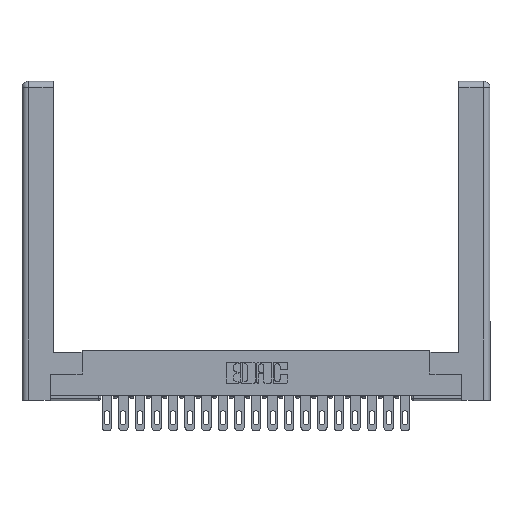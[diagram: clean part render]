
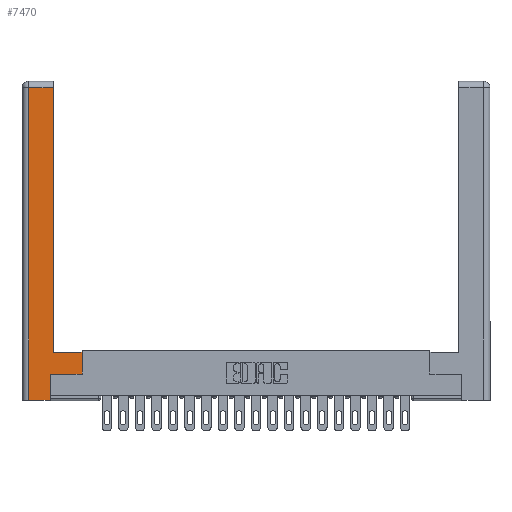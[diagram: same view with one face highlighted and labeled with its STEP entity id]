
A CAD part, top view. The second image highlights one B-rep face of the part: STEP entity #7470.
In plain terms, the highlighted planar face has unit normal (0, 0, 1).
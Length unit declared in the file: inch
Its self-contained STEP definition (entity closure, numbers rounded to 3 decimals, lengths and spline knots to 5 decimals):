
#186 = VECTOR ( 'NONE', #10621, 39.37008 ) ;
#379 = VERTEX_POINT ( 'NONE', #3913 ) ;
#973 = DIRECTION ( 'NONE',  ( 1., 0., 0. ) ) ;
#1471 = DIRECTION ( 'NONE',  ( 1., 0., 0. ) ) ;
#2467 = CARTESIAN_POINT ( 'NONE',  ( 0.565, 0.245, 0. ) ) ;
#2537 = CARTESIAN_POINT ( 'NONE',  ( 0.295, 0.45, 0. ) ) ;
#2894 = ORIENTED_EDGE ( 'NONE', *, *, #5513, .T. ) ;
#3110 = VERTEX_POINT ( 'NONE', #10268 ) ;
#3639 = EDGE_CURVE ( 'NONE', #11047, #18683, #11877, .T. ) ;
#3889 = ORIENTED_EDGE ( 'NONE', *, *, #11764, .T. ) ;
#3912 = LINE ( 'NONE', #11777, #4987 ) ;
#3913 = CARTESIAN_POINT ( 'NONE',  ( 0.565, 0.245, 0. ) ) ;
#4777 = LINE ( 'NONE', #17486, #186 ) ;
#4929 = CARTESIAN_POINT ( 'NONE',  ( 0.565, 0.45, 0. ) ) ;
#4987 = VECTOR ( 'NONE', #13515, 39.37008 ) ;
#5513 = EDGE_CURVE ( 'NONE', #15409, #9972, #21355, .T. ) ;
#7267 = VECTOR ( 'NONE', #15089, 39.37008 ) ;
#7470 = ADVANCED_FACE ( 'NONE', ( #11605 ), #15711, .F. ) ;
#7806 = VECTOR ( 'NONE', #973, 39.37008 ) ;
#8087 = CARTESIAN_POINT ( 'NONE',  ( 0.265, 0.245, 0. ) ) ;
#8167 = LINE ( 'NONE', #4929, #21642 ) ;
#8504 = VERTEX_POINT ( 'NONE', #21378 ) ;
#8643 = CARTESIAN_POINT ( 'NONE',  ( 0., 0., 0. ) ) ;
#9398 = LINE ( 'NONE', #14308, #13458 ) ;
#9646 = EDGE_CURVE ( 'NONE', #3110, #9737, #9398, .T. ) ;
#9737 = VERTEX_POINT ( 'NONE', #2537 ) ;
#9922 = EDGE_LOOP ( 'NONE', ( #20953, #2894, #3889, #19506, #21054, #11609, #11602, #10057 ) ) ;
#9972 = VERTEX_POINT ( 'NONE', #13472 ) ;
#10057 = ORIENTED_EDGE ( 'NONE', *, *, #9646, .T. ) ;
#10268 = CARTESIAN_POINT ( 'NONE',  ( 0.565, 0.45, 0. ) ) ;
#10621 = DIRECTION ( 'NONE',  ( 0., 1., 0. ) ) ;
#11047 = VERTEX_POINT ( 'NONE', #16432 ) ;
#11336 = AXIS2_PLACEMENT_3D ( 'NONE', #8643, #20630, #18810 ) ;
#11602 = ORIENTED_EDGE ( 'NONE', *, *, #16016, .T. ) ;
#11605 = FACE_OUTER_BOUND ( 'NONE', #9922, .T. ) ;
#11609 = ORIENTED_EDGE ( 'NONE', *, *, #18505, .T. ) ;
#11764 = EDGE_CURVE ( 'NONE', #9972, #8504, #3912, .T. ) ;
#11777 = CARTESIAN_POINT ( 'NONE',  ( 0.0615, 0., 0. ) ) ;
#11877 = LINE ( 'NONE', #8087, #7267 ) ;
#13286 = VECTOR ( 'NONE', #19680, 39.37008 ) ;
#13458 = VECTOR ( 'NONE', #14521, 39.37008 ) ;
#13472 = CARTESIAN_POINT ( 'NONE',  ( 0.0615, 2.94, 0. ) ) ;
#13515 = DIRECTION ( 'NONE',  ( 0., -1., 0. ) ) ;
#14003 = CARTESIAN_POINT ( 'NONE',  ( 0.265, 0.245, 0. ) ) ;
#14308 = CARTESIAN_POINT ( 'NONE',  ( 0.295, 0.45, 0. ) ) ;
#14521 = DIRECTION ( 'NONE',  ( -1., 0., 0. ) ) ;
#15089 = DIRECTION ( 'NONE',  ( 0., 1., 0. ) ) ;
#15289 = CARTESIAN_POINT ( 'NONE',  ( 0.295, 2.94, 0. ) ) ;
#15397 = EDGE_CURVE ( 'NONE', #8504, #11047, #21124, .T. ) ;
#15409 = VERTEX_POINT ( 'NONE', #15289 ) ;
#15711 = PLANE ( 'NONE',  #11336 ) ;
#16016 = EDGE_CURVE ( 'NONE', #379, #3110, #8167, .T. ) ;
#16432 = CARTESIAN_POINT ( 'NONE',  ( 0.265, 0., 0. ) ) ;
#17486 = CARTESIAN_POINT ( 'NONE',  ( 0.295, 3., 0. ) ) ;
#17515 = LINE ( 'NONE', #2467, #7806 ) ;
#18505 = EDGE_CURVE ( 'NONE', #18683, #379, #17515, .T. ) ;
#18683 = VERTEX_POINT ( 'NONE', #14003 ) ;
#18754 = CARTESIAN_POINT ( 'NONE',  ( 0.265, 0., 0. ) ) ;
#18810 = DIRECTION ( 'NONE',  ( -1., 0., 0. ) ) ;
#19506 = ORIENTED_EDGE ( 'NONE', *, *, #15397, .T. ) ;
#19680 = DIRECTION ( 'NONE',  ( -1., 0., 0. ) ) ;
#19858 = CARTESIAN_POINT ( 'NONE',  ( 0.0615, 2.94, 0. ) ) ;
#20031 = EDGE_CURVE ( 'NONE', #9737, #15409, #4777, .T. ) ;
#20630 = DIRECTION ( 'NONE',  ( 0., 0., -1. ) ) ;
#20694 = DIRECTION ( 'NONE',  ( 0., 1., 0. ) ) ;
#20953 = ORIENTED_EDGE ( 'NONE', *, *, #20031, .T. ) ;
#21054 = ORIENTED_EDGE ( 'NONE', *, *, #3639, .T. ) ;
#21124 = LINE ( 'NONE', #18754, #22221 ) ;
#21355 = LINE ( 'NONE', #19858, #13286 ) ;
#21378 = CARTESIAN_POINT ( 'NONE',  ( 0.0615, 0., 0. ) ) ;
#21642 = VECTOR ( 'NONE', #20694, 39.37008 ) ;
#22221 = VECTOR ( 'NONE', #1471, 39.37008 ) ;
